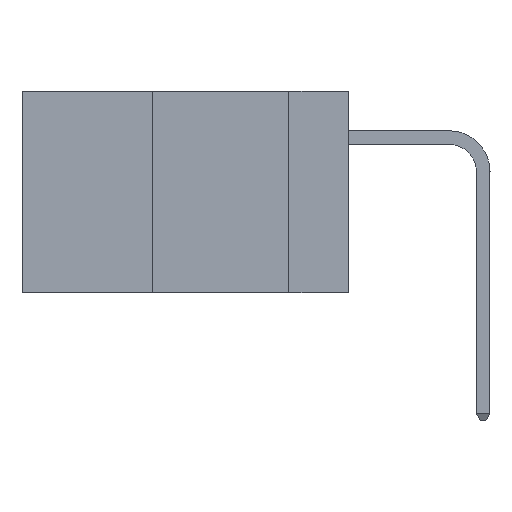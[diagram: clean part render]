
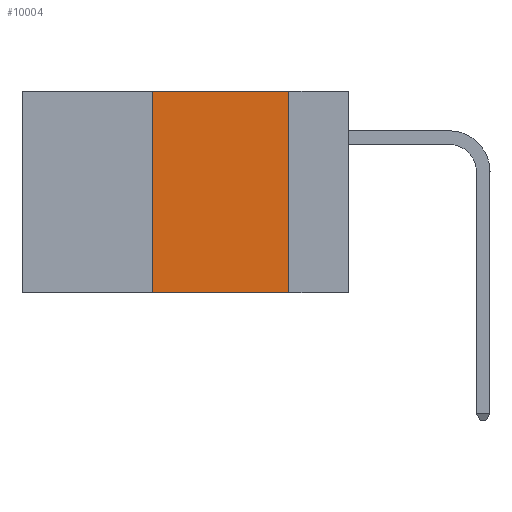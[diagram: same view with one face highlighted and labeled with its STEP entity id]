
A CAD part, left-side view. The second image highlights one B-rep face of the part: STEP entity #10004.
In plain terms, the highlighted planar face has unit normal (-1, 0, 0).
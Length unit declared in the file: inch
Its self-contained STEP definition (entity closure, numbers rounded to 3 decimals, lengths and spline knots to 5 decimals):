
#14 = ORIENTED_EDGE ( 'NONE', *, *, #193, .F. ) ;
#193 = EDGE_CURVE ( 'NONE', #23774, #8466, #17751, .T. ) ;
#535 = EDGE_CURVE ( 'NONE', #23774, #7127, #4985, .T. ) ;
#767 = DIRECTION ( 'NONE',  ( 0., -1., 0. ) ) ;
#2050 = VECTOR ( 'NONE', #5912, 39.37008 ) ;
#2164 = DIRECTION ( 'NONE',  ( 0., -1., 0. ) ) ;
#2690 = LINE ( 'NONE', #15840, #2050 ) ;
#2873 = CARTESIAN_POINT ( 'NONE',  ( 0., 0.6, -0.37 ) ) ;
#2976 = FACE_OUTER_BOUND ( 'NONE', #25537, .T. ) ;
#3573 = AXIS2_PLACEMENT_3D ( 'NONE', #14066, #6140, #20056 ) ;
#4067 = PLANE ( 'NONE',  #3573 ) ;
#4842 = VECTOR ( 'NONE', #767, 39.37008 ) ;
#4985 = LINE ( 'NONE', #2873, #20214 ) ;
#5624 = CARTESIAN_POINT ( 'NONE',  ( 0., 0.36, 0. ) ) ;
#5912 = DIRECTION ( 'NONE',  ( 0., 0., -1. ) ) ;
#6140 = DIRECTION ( 'NONE',  ( 1., 0., 0. ) ) ;
#6343 = ORIENTED_EDGE ( 'NONE', *, *, #535, .T. ) ;
#7127 = VERTEX_POINT ( 'NONE', #20560 ) ;
#8466 = VERTEX_POINT ( 'NONE', #10929 ) ;
#9407 = EDGE_CURVE ( 'NONE', #16803, #7127, #2690, .T. ) ;
#9985 = CARTESIAN_POINT ( 'NONE',  ( 0., 0.36, -0.37 ) ) ;
#10004 = ADVANCED_FACE ( 'NONE', ( #2976 ), #4067, .F. ) ;
#10766 = CARTESIAN_POINT ( 'NONE',  ( 0., 0.6, 0. ) ) ;
#10929 = CARTESIAN_POINT ( 'NONE',  ( 0., 0.36, 0. ) ) ;
#12294 = CARTESIAN_POINT ( 'NONE',  ( 0., 0.11, 0. ) ) ;
#13532 = ORIENTED_EDGE ( 'NONE', *, *, #9407, .F. ) ;
#14066 = CARTESIAN_POINT ( 'NONE',  ( 0., 0.6, 0. ) ) ;
#15437 = LINE ( 'NONE', #10766, #4842 ) ;
#15546 = EDGE_CURVE ( 'NONE', #8466, #16803, #15437, .T. ) ;
#15840 = CARTESIAN_POINT ( 'NONE',  ( 0., 0.11, 0. ) ) ;
#16803 = VERTEX_POINT ( 'NONE', #12294 ) ;
#17751 = LINE ( 'NONE', #5624, #22946 ) ;
#17947 = ORIENTED_EDGE ( 'NONE', *, *, #15546, .F. ) ;
#19177 = DIRECTION ( 'NONE',  ( 0., 0., 1. ) ) ;
#20056 = DIRECTION ( 'NONE',  ( 0., 0., -1. ) ) ;
#20214 = VECTOR ( 'NONE', #2164, 39.37008 ) ;
#20560 = CARTESIAN_POINT ( 'NONE',  ( 0., 0.11, -0.37 ) ) ;
#22946 = VECTOR ( 'NONE', #19177, 39.37008 ) ;
#23774 = VERTEX_POINT ( 'NONE', #9985 ) ;
#25537 = EDGE_LOOP ( 'NONE', ( #13532, #17947, #14, #6343 ) ) ;
